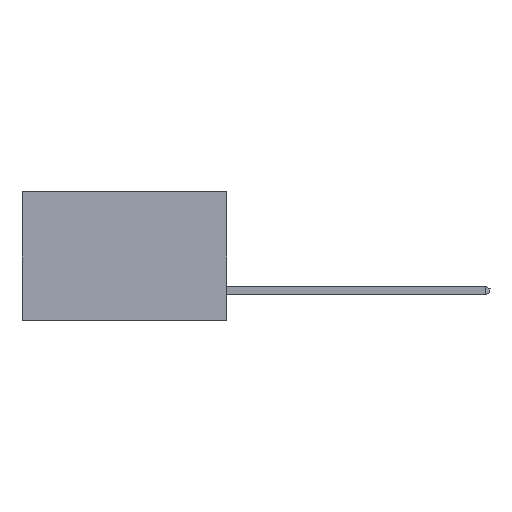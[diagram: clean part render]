
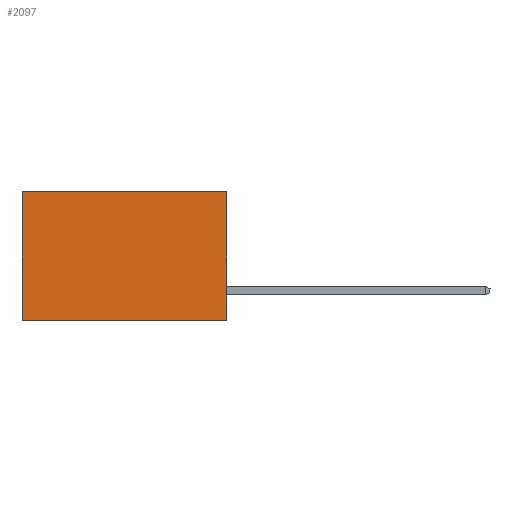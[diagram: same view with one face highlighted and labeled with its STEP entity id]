
A CAD part, left-side view. The second image highlights one B-rep face of the part: STEP entity #2097.
In plain terms, the highlighted planar face has unit normal (-1, 0, 0).
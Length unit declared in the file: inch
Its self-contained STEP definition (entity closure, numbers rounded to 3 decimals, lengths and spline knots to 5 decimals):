
#164 = LINE ( 'NONE', #10220, #12628 ) ;
#945 = LINE ( 'NONE', #4708, #12263 ) ;
#1187 = VERTEX_POINT ( 'NONE', #1622 ) ;
#1284 = EDGE_CURVE ( 'NONE', #11433, #1187, #2211, .T. ) ;
#1622 = CARTESIAN_POINT ( 'NONE',  ( 0.277, 0.59, -0.37 ) ) ;
#2097 = ADVANCED_FACE ( 'NONE', ( #3617 ), #4123, .F. ) ;
#2211 = LINE ( 'NONE', #5970, #4886 ) ;
#3024 = DIRECTION ( 'NONE',  ( 0., 0., -1. ) ) ;
#3617 = FACE_OUTER_BOUND ( 'NONE', #10730, .T. ) ;
#4037 = CARTESIAN_POINT ( 'NONE',  ( 0.277, 0., 0. ) ) ;
#4123 = PLANE ( 'NONE',  #5319 ) ;
#4585 = DIRECTION ( 'NONE',  ( 0., 1., 0. ) ) ;
#4666 = CARTESIAN_POINT ( 'NONE',  ( 0.277, 0.59, 0. ) ) ;
#4708 = CARTESIAN_POINT ( 'NONE',  ( 0.277, 0., -0.37 ) ) ;
#4886 = VECTOR ( 'NONE', #3024, 39.37008 ) ;
#5049 = DIRECTION ( 'NONE',  ( 0., 0., -1. ) ) ;
#5186 = DIRECTION ( 'NONE',  ( 1., 0., 0. ) ) ;
#5319 = AXIS2_PLACEMENT_3D ( 'NONE', #10982, #5186, #5049 ) ;
#5690 = ORIENTED_EDGE ( 'NONE', *, *, #8532, .T. ) ;
#5970 = CARTESIAN_POINT ( 'NONE',  ( 0.277, 0.59, -0.37 ) ) ;
#6510 = LINE ( 'NONE', #4037, #9062 ) ;
#6513 = VERTEX_POINT ( 'NONE', #13527 ) ;
#6563 = EDGE_CURVE ( 'NONE', #6513, #10674, #164, .T. ) ;
#7426 = ORIENTED_EDGE ( 'NONE', *, *, #7486, .F. ) ;
#7486 = EDGE_CURVE ( 'NONE', #10674, #1187, #945, .T. ) ;
#8532 = EDGE_CURVE ( 'NONE', #6513, #11433, #6510, .T. ) ;
#9062 = VECTOR ( 'NONE', #11858, 39.37008 ) ;
#10220 = CARTESIAN_POINT ( 'NONE',  ( 0.277, 0., -0.37 ) ) ;
#10281 = DIRECTION ( 'NONE',  ( 0., 0., -1. ) ) ;
#10336 = ORIENTED_EDGE ( 'NONE', *, *, #6563, .F. ) ;
#10674 = VERTEX_POINT ( 'NONE', #13662 ) ;
#10730 = EDGE_LOOP ( 'NONE', ( #14308, #7426, #10336, #5690 ) ) ;
#10982 = CARTESIAN_POINT ( 'NONE',  ( 0.277, 0., -0.37 ) ) ;
#11433 = VERTEX_POINT ( 'NONE', #4666 ) ;
#11858 = DIRECTION ( 'NONE',  ( 0., 1., 0. ) ) ;
#12263 = VECTOR ( 'NONE', #4585, 39.37008 ) ;
#12628 = VECTOR ( 'NONE', #10281, 39.37008 ) ;
#13527 = CARTESIAN_POINT ( 'NONE',  ( 0.277, 0., 0. ) ) ;
#13662 = CARTESIAN_POINT ( 'NONE',  ( 0.277, 0., -0.37 ) ) ;
#14308 = ORIENTED_EDGE ( 'NONE', *, *, #1284, .T. ) ;
